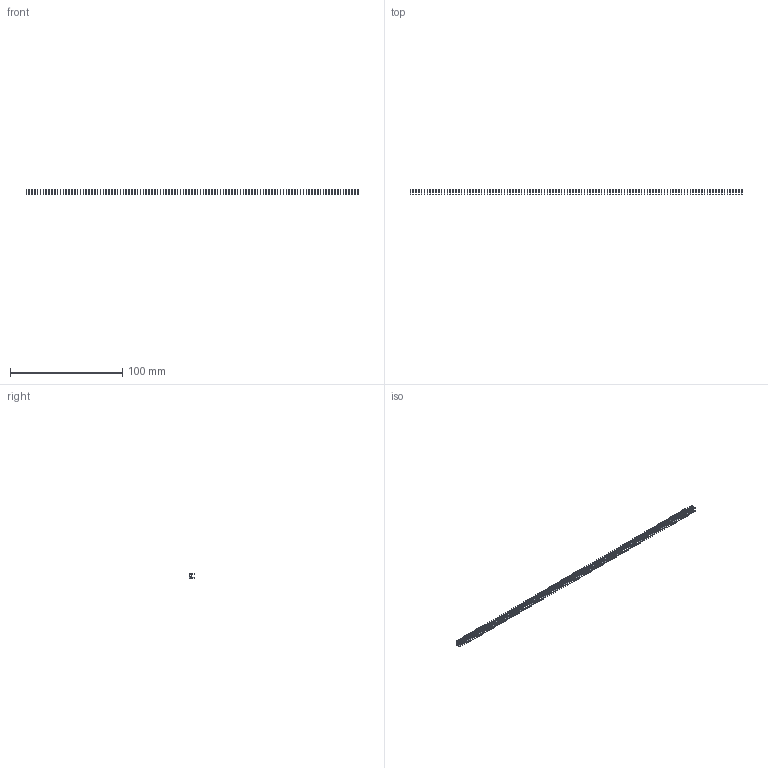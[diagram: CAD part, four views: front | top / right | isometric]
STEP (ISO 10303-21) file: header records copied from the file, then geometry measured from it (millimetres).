
FILE_DESCRIPTION (( 'STEP AP203' ), '1' );
FILE_NAME ('105-117-208-100.STEP', '2020-04-08T01:26:13', ( '' ), ( '' ), 'SwSTEP 2.0', 'SolidWorks 2016', '' );
FILE_SCHEMA (( 'CONFIG_CONTROL_DESIGN' ));
Length unit declared in the file: inch
Products named in the file (2): 105-117-208-100; 100-290-001_100-290-208
Assembly tree (117 placements, depth 2):
  105-117-208-100
    100-290-001_100-290-208  x117
Bounding box: 295.15 x 4.83 x 5.17 mm (x, y, z)
Volume: 805 mm3; surface area: 4972 mm2
Topology: 117 solids, 117 shells, 2925 faces, 8073 edges, 5382 vertices
Faces by surface type: plane 2574, cylinder 351
Entity records: 4701 total; most frequent: DIRECTION 365, CARTESIAN_POINT 260, CALENDAR_DATE 244, DATE_AND_TIME 244, COORDINATED_UNIVERSAL_TIME_OFFSET 244, LOCAL_TIME 244, AXIS2_PLACEMENT_3D 151, ORIENTED_EDGE 138
